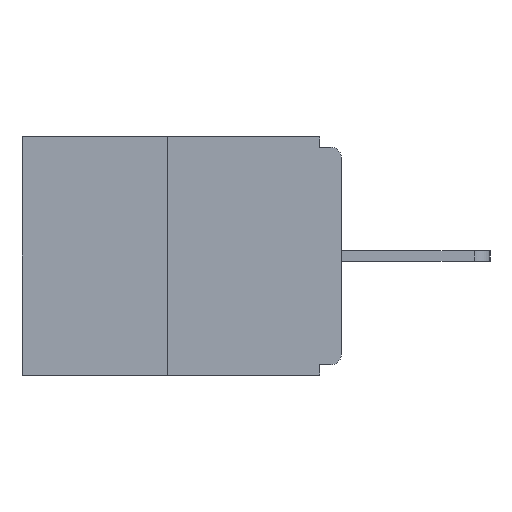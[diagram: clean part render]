
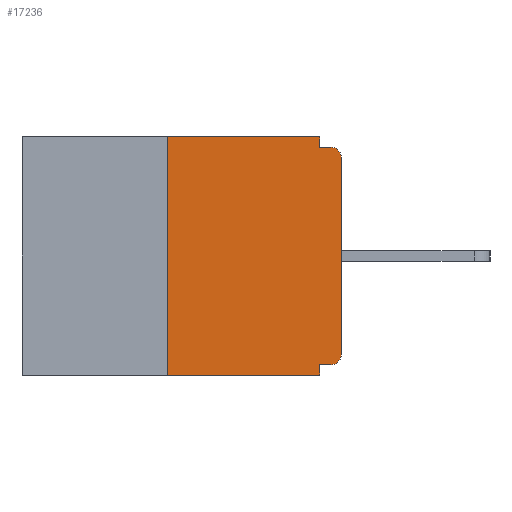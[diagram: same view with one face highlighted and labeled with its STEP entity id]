
A CAD part, left-side view. The second image highlights one B-rep face of the part: STEP entity #17236.
In plain terms, the highlighted planar face has unit normal (-1, 0, 0).
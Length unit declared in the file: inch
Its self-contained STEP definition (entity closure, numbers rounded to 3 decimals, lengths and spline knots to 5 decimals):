
#27 = EDGE_CURVE ( 'NONE', #12698, #1767, #6938, .T. ) ;
#441 = VECTOR ( 'NONE', #18362, 39.37008 ) ;
#487 = VERTEX_POINT ( 'NONE', #4326 ) ;
#786 = VECTOR ( 'NONE', #13340, 39.37008 ) ;
#821 = CARTESIAN_POINT ( 'NONE',  ( 0., 0., -0.313 ) ) ;
#1009 = DIRECTION ( 'NONE',  ( 0., 0., -1. ) ) ;
#1105 = LINE ( 'NONE', #14910, #14761 ) ;
#1206 = DIRECTION ( 'NONE',  ( 0., 0., -1. ) ) ;
#1211 = CARTESIAN_POINT ( 'NONE',  ( 0., 0.46, 0. ) ) ;
#1231 = EDGE_CURVE ( 'NONE', #17763, #487, #19991, .T. ) ;
#1281 = EDGE_CURVE ( 'NONE', #22231, #17763, #1105, .T. ) ;
#1402 = ORIENTED_EDGE ( 'NONE', *, *, #18909, .T. ) ;
#1636 = ORIENTED_EDGE ( 'NONE', *, *, #16026, .F. ) ;
#1767 = VERTEX_POINT ( 'NONE', #15529 ) ;
#2287 = CARTESIAN_POINT ( 'NONE',  ( 0., 0.25, 0. ) ) ;
#3104 = DIRECTION ( 'NONE',  ( -1., 0., 0. ) ) ;
#3379 = ORIENTED_EDGE ( 'NONE', *, *, #27, .F. ) ;
#3446 = CARTESIAN_POINT ( 'NONE',  ( 0., 0.015, -0.03 ) ) ;
#3474 = CARTESIAN_POINT ( 'NONE',  ( 0., 0., -0.328 ) ) ;
#3484 = CARTESIAN_POINT ( 'NONE',  ( 0., 0.25, -0.343 ) ) ;
#3686 = DIRECTION ( 'NONE',  ( 0., 1., 0. ) ) ;
#3798 = EDGE_CURVE ( 'NONE', #17863, #4616, #18535, .T. ) ;
#4008 = AXIS2_PLACEMENT_3D ( 'NONE', #18765, #6490, #9987 ) ;
#4326 = CARTESIAN_POINT ( 'NONE',  ( 0., 0.031, 0. ) ) ;
#4616 = VERTEX_POINT ( 'NONE', #21989 ) ;
#4764 = ORIENTED_EDGE ( 'NONE', *, *, #9240, .T. ) ;
#5025 = CARTESIAN_POINT ( 'NONE',  ( 0., 0., -0.015 ) ) ;
#5533 = CARTESIAN_POINT ( 'NONE',  ( 0., 0.015, -0.313 ) ) ;
#6383 = LINE ( 'NONE', #20118, #11578 ) ;
#6490 = DIRECTION ( 'NONE',  ( 1., 0., 0. ) ) ;
#6768 = EDGE_LOOP ( 'NONE', ( #19471, #20806, #4764, #9578, #3379, #7334, #16524, #1402, #19802, #1636 ) ) ;
#6938 = LINE ( 'NONE', #3474, #6981 ) ;
#6981 = VECTOR ( 'NONE', #3686, 39.37008 ) ;
#7334 = ORIENTED_EDGE ( 'NONE', *, *, #10379, .T. ) ;
#7663 = CIRCLE ( 'NONE', #20258, 0.015 ) ;
#7797 = LINE ( 'NONE', #11506, #441 ) ;
#7879 = CARTESIAN_POINT ( 'NONE',  ( 0., 0.031, -0.015 ) ) ;
#8098 = LINE ( 'NONE', #16204, #8158 ) ;
#8158 = VECTOR ( 'NONE', #14844, 39.37008 ) ;
#8195 = CIRCLE ( 'NONE', #10737, 0.015 ) ;
#8353 = VECTOR ( 'NONE', #22188, 39.37008 ) ;
#9240 = EDGE_CURVE ( 'NONE', #22231, #10258, #8098, .T. ) ;
#9578 = ORIENTED_EDGE ( 'NONE', *, *, #16306, .F. ) ;
#9687 = VERTEX_POINT ( 'NONE', #16402 ) ;
#9987 = DIRECTION ( 'NONE',  ( 0., 0., -1. ) ) ;
#10011 = CARTESIAN_POINT ( 'NONE',  ( 0., 0.031, 0. ) ) ;
#10258 = VERTEX_POINT ( 'NONE', #21997 ) ;
#10379 = EDGE_CURVE ( 'NONE', #12698, #11669, #8195, .T. ) ;
#10737 = AXIS2_PLACEMENT_3D ( 'NONE', #5533, #17680, #15663 ) ;
#11506 = CARTESIAN_POINT ( 'NONE',  ( 0., 0., 0. ) ) ;
#11578 = VECTOR ( 'NONE', #1009, 39.37008 ) ;
#11669 = VERTEX_POINT ( 'NONE', #821 ) ;
#11780 = CARTESIAN_POINT ( 'NONE',  ( 0., 0.015, -0.328 ) ) ;
#12698 = VERTEX_POINT ( 'NONE', #11780 ) ;
#13340 = DIRECTION ( 'NONE',  ( 0., -1., 0. ) ) ;
#14248 = VECTOR ( 'NONE', #21716, 39.37008 ) ;
#14761 = VECTOR ( 'NONE', #18079, 39.37008 ) ;
#14844 = DIRECTION ( 'NONE',  ( 0., -1., 0. ) ) ;
#14910 = CARTESIAN_POINT ( 'NONE',  ( 0., 0.25, 0. ) ) ;
#15289 = LINE ( 'NONE', #10011, #8353 ) ;
#15498 = EDGE_CURVE ( 'NONE', #11669, #9687, #7797, .T. ) ;
#15529 = CARTESIAN_POINT ( 'NONE',  ( 0., 0.031, -0.328 ) ) ;
#15663 = DIRECTION ( 'NONE',  ( 0., 0., -1. ) ) ;
#16026 = EDGE_CURVE ( 'NONE', #487, #17863, #15289, .T. ) ;
#16204 = CARTESIAN_POINT ( 'NONE',  ( 0., 0.46, -0.343 ) ) ;
#16306 = EDGE_CURVE ( 'NONE', #1767, #10258, #6383, .T. ) ;
#16402 = CARTESIAN_POINT ( 'NONE',  ( 0., 0., -0.03 ) ) ;
#16524 = ORIENTED_EDGE ( 'NONE', *, *, #15498, .T. ) ;
#17236 = ADVANCED_FACE ( 'NONE', ( #20235 ), #20352, .F. ) ;
#17680 = DIRECTION ( 'NONE',  ( -1., 0., 0. ) ) ;
#17763 = VERTEX_POINT ( 'NONE', #2287 ) ;
#17863 = VERTEX_POINT ( 'NONE', #7879 ) ;
#18079 = DIRECTION ( 'NONE',  ( 0., 0., 1. ) ) ;
#18362 = DIRECTION ( 'NONE',  ( 0., 0., 1. ) ) ;
#18535 = LINE ( 'NONE', #5025, #14248 ) ;
#18765 = CARTESIAN_POINT ( 'NONE',  ( 0., 0.46, 0. ) ) ;
#18909 = EDGE_CURVE ( 'NONE', #9687, #4616, #7663, .T. ) ;
#19471 = ORIENTED_EDGE ( 'NONE', *, *, #1231, .F. ) ;
#19802 = ORIENTED_EDGE ( 'NONE', *, *, #3798, .F. ) ;
#19991 = LINE ( 'NONE', #1211, #786 ) ;
#20118 = CARTESIAN_POINT ( 'NONE',  ( 0., 0.031, -0.343 ) ) ;
#20235 = FACE_OUTER_BOUND ( 'NONE', #6768, .T. ) ;
#20258 = AXIS2_PLACEMENT_3D ( 'NONE', #3446, #3104, #1206 ) ;
#20352 = PLANE ( 'NONE',  #4008 ) ;
#20806 = ORIENTED_EDGE ( 'NONE', *, *, #1281, .F. ) ;
#21716 = DIRECTION ( 'NONE',  ( 0., -1., 0. ) ) ;
#21989 = CARTESIAN_POINT ( 'NONE',  ( 0., 0.015, -0.015 ) ) ;
#21997 = CARTESIAN_POINT ( 'NONE',  ( 0., 0.031, -0.343 ) ) ;
#22188 = DIRECTION ( 'NONE',  ( 0., 0., -1. ) ) ;
#22231 = VERTEX_POINT ( 'NONE', #3484 ) ;
